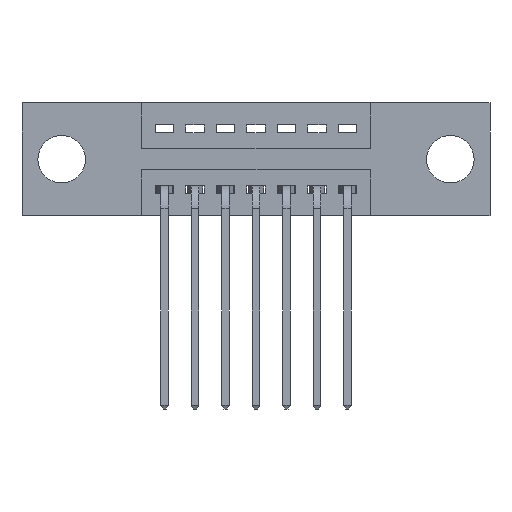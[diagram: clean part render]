
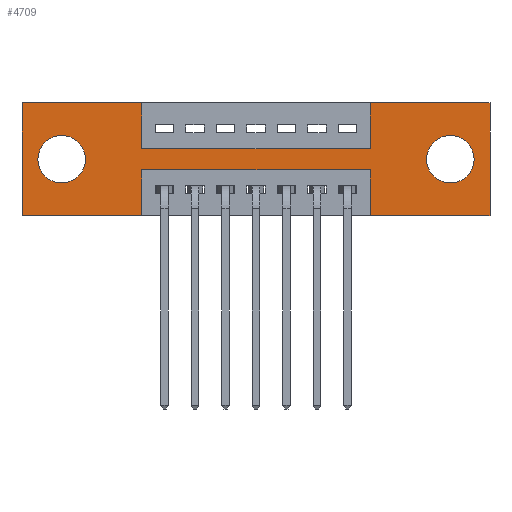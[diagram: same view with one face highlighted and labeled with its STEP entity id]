
A CAD part, front view. The second image highlights one B-rep face of the part: STEP entity #4709.
In plain terms, the highlighted planar face has unit normal (0, -1, 0).
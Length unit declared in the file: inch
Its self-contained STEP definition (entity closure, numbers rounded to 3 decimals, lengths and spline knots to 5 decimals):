
#4 = DIRECTION ( 'NONE',  ( 0., 0., 1. ) ) ;
#67 = ORIENTED_EDGE ( 'NONE', *, *, #2431, .F. ) ;
#70 = ORIENTED_EDGE ( 'NONE', *, *, #4872, .F. ) ;
#92 = ORIENTED_EDGE ( 'NONE', *, *, #8722, .F. ) ;
#132 = ORIENTED_EDGE ( 'NONE', *, *, #4977, .T. ) ;
#203 = ORIENTED_EDGE ( 'NONE', *, *, #1343, .F. ) ;
#391 = ORIENTED_EDGE ( 'NONE', *, *, #4073, .F. ) ;
#434 = CARTESIAN_POINT ( 'NONE',  ( 1.405, 0., -0.107 ) ) ;
#557 = ORIENTED_EDGE ( 'NONE', *, *, #3080, .T. ) ;
#597 = VERTEX_POINT ( 'NONE', #6072 ) ;
#625 = EDGE_CURVE ( 'NONE', #7750, #8362, #4138, .T. ) ;
#644 = VERTEX_POINT ( 'NONE', #993 ) ;
#658 = ORIENTED_EDGE ( 'NONE', *, *, #10028, .F. ) ;
#693 = CARTESIAN_POINT ( 'NONE',  ( 0., 0., -0.37 ) ) ;
#799 = VERTEX_POINT ( 'NONE', #434 ) ;
#810 = EDGE_CURVE ( 'NONE', #5263, #7720, #3069, .T. ) ;
#854 = CARTESIAN_POINT ( 'NONE',  ( 0.13, 0., -0.107 ) ) ;
#937 = VECTOR ( 'NONE', #6131, 39.37008 ) ;
#993 = CARTESIAN_POINT ( 'NONE',  ( 0.3925, 0., -0.37 ) ) ;
#1066 = VECTOR ( 'NONE', #4671, 39.37008 ) ;
#1343 = EDGE_CURVE ( 'NONE', #9410, #3716, #3558, .T. ) ;
#1416 = FACE_OUTER_BOUND ( 'NONE', #4132, .T. ) ;
#1428 = ORIENTED_EDGE ( 'NONE', *, *, #3376, .T. ) ;
#1438 = ORIENTED_EDGE ( 'NONE', *, *, #625, .F. ) ;
#1467 = DIRECTION ( 'NONE',  ( 0., 0., -1. ) ) ;
#1473 = DIRECTION ( 'NONE',  ( 0., 1., 0. ) ) ;
#1483 = CARTESIAN_POINT ( 'NONE',  ( 1.405, 0., -0.185 ) ) ;
#1587 = CARTESIAN_POINT ( 'NONE',  ( 1.535, 0., 0. ) ) ;
#1611 = CARTESIAN_POINT ( 'NONE',  ( 0., 0., -0.37 ) ) ;
#1643 = VERTEX_POINT ( 'NONE', #693 ) ;
#1645 = DIRECTION ( 'NONE',  ( 0., 1., 0. ) ) ;
#1715 = CARTESIAN_POINT ( 'NONE',  ( 0., 0., -0.37 ) ) ;
#1917 = VECTOR ( 'NONE', #8969, 39.37008 ) ;
#2101 = VECTOR ( 'NONE', #2551, 39.37008 ) ;
#2142 = CIRCLE ( 'NONE', #7641, 0.078 ) ;
#2307 = ORIENTED_EDGE ( 'NONE', *, *, #810, .T. ) ;
#2379 = CARTESIAN_POINT ( 'NONE',  ( 0.3925, 0., 0. ) ) ;
#2431 = EDGE_CURVE ( 'NONE', #5848, #7120, #4400, .T. ) ;
#2453 = DIRECTION ( 'NONE',  ( -1., 0., 0. ) ) ;
#2533 = AXIS2_PLACEMENT_3D ( 'NONE', #3192, #3287, #3289 ) ;
#2551 = DIRECTION ( 'NONE',  ( 0., 0., -1. ) ) ;
#2730 = ORIENTED_EDGE ( 'NONE', *, *, #9219, .F. ) ;
#2784 = CIRCLE ( 'NONE', #2533, 0.078 ) ;
#2812 = ORIENTED_EDGE ( 'NONE', *, *, #6426, .F. ) ;
#2928 = ORIENTED_EDGE ( 'NONE', *, *, #8620, .F. ) ;
#3069 = CIRCLE ( 'NONE', #7272, 0.078 ) ;
#3080 = EDGE_CURVE ( 'NONE', #799, #597, #2784, .T. ) ;
#3160 = DIRECTION ( 'NONE',  ( 1., 0., 0. ) ) ;
#3192 = CARTESIAN_POINT ( 'NONE',  ( 1.405, 0., -0.185 ) ) ;
#3262 = LINE ( 'NONE', #9622, #1066 ) ;
#3287 = DIRECTION ( 'NONE',  ( 0., 1., 0. ) ) ;
#3289 = DIRECTION ( 'NONE',  ( 0., 0., -1. ) ) ;
#3376 = EDGE_CURVE ( 'NONE', #7720, #5263, #2142, .T. ) ;
#3449 = DIRECTION ( 'NONE',  ( 0., 0., -1. ) ) ;
#3458 = PLANE ( 'NONE',  #8005 ) ;
#3483 = CARTESIAN_POINT ( 'NONE',  ( 0., 0., -0.37 ) ) ;
#3550 = DIRECTION ( 'NONE',  ( 0., -1., 0. ) ) ;
#3558 = LINE ( 'NONE', #6104, #9057 ) ;
#3716 = VERTEX_POINT ( 'NONE', #4149 ) ;
#3879 = FACE_BOUND ( 'NONE', #3880, .T. ) ;
#3880 = EDGE_LOOP ( 'NONE', ( #557, #132 ) ) ;
#4000 = CARTESIAN_POINT ( 'NONE',  ( 0.3925, 0., -0.15 ) ) ;
#4073 = EDGE_CURVE ( 'NONE', #8362, #644, #9103, .T. ) ;
#4132 = EDGE_LOOP ( 'NONE', ( #391, #1438, #92, #8539, #2730, #67, #8314, #2812, #70, #203, #2928, #658 ) ) ;
#4138 = LINE ( 'NONE', #4354, #1917 ) ;
#4149 = CARTESIAN_POINT ( 'NONE',  ( 0.3925, 0., 0. ) ) ;
#4186 = EDGE_LOOP ( 'NONE', ( #2307, #1428 ) ) ;
#4230 = CARTESIAN_POINT ( 'NONE',  ( 1.1425, 0., 0. ) ) ;
#4323 = VECTOR ( 'NONE', #3160, 39.37008 ) ;
#4354 = CARTESIAN_POINT ( 'NONE',  ( 0.3925, 0., -0.22 ) ) ;
#4400 = LINE ( 'NONE', #6595, #9681 ) ;
#4671 = DIRECTION ( 'NONE',  ( 0., 0., -1. ) ) ;
#4709 = ADVANCED_FACE ( 'NONE', ( #3879, #6087, #1416 ), #3458, .T. ) ;
#4872 = EDGE_CURVE ( 'NONE', #3716, #9176, #8280, .T. ) ;
#4911 = CARTESIAN_POINT ( 'NONE',  ( 0., 0., 0. ) ) ;
#4977 = EDGE_CURVE ( 'NONE', #597, #799, #7218, .T. ) ;
#5263 = VERTEX_POINT ( 'NONE', #854 ) ;
#5353 = CARTESIAN_POINT ( 'NONE',  ( 0., 0., 0. ) ) ;
#5410 = CARTESIAN_POINT ( 'NONE',  ( 0.3925, 0., -0.15 ) ) ;
#5416 = LINE ( 'NONE', #5353, #937 ) ;
#5535 = DIRECTION ( 'NONE',  ( 1., 0., 0. ) ) ;
#5761 = CARTESIAN_POINT ( 'NONE',  ( 0.13, 0., -0.263 ) ) ;
#5792 = CARTESIAN_POINT ( 'NONE',  ( 0.3925, 0., -0.22 ) ) ;
#5848 = VERTEX_POINT ( 'NONE', #4230 ) ;
#5990 = CARTESIAN_POINT ( 'NONE',  ( 1.1425, 0., -0.15 ) ) ;
#5991 = VERTEX_POINT ( 'NONE', #5990 ) ;
#6072 = CARTESIAN_POINT ( 'NONE',  ( 1.405, 0., -0.263 ) ) ;
#6087 = FACE_BOUND ( 'NONE', #4186, .T. ) ;
#6104 = CARTESIAN_POINT ( 'NONE',  ( 0., 0., 0. ) ) ;
#6131 = DIRECTION ( 'NONE',  ( 0., 0., 1. ) ) ;
#6154 = DIRECTION ( 'NONE',  ( 1., 0., 0. ) ) ;
#6426 = EDGE_CURVE ( 'NONE', #9176, #5991, #10036, .T. ) ;
#6427 = AXIS2_PLACEMENT_3D ( 'NONE', #1483, #1473, #1467 ) ;
#6477 = VECTOR ( 'NONE', #8400, 39.37008 ) ;
#6595 = CARTESIAN_POINT ( 'NONE',  ( 0., 0., 0. ) ) ;
#6710 = LINE ( 'NONE', #9605, #6477 ) ;
#7120 = VERTEX_POINT ( 'NONE', #1587 ) ;
#7218 = CIRCLE ( 'NONE', #6427, 0.078 ) ;
#7272 = AXIS2_PLACEMENT_3D ( 'NONE', #9118, #1645, #4 ) ;
#7276 = CARTESIAN_POINT ( 'NONE',  ( 1.535, 0., -0.37 ) ) ;
#7330 = DIRECTION ( 'NONE',  ( -1., 0., 0. ) ) ;
#7362 = VECTOR ( 'NONE', #9241, 39.37008 ) ;
#7411 = VECTOR ( 'NONE', #8667, 39.37008 ) ;
#7584 = CARTESIAN_POINT ( 'NONE',  ( 1.1425, 0., -0.37 ) ) ;
#7627 = LINE ( 'NONE', #10021, #7411 ) ;
#7641 = AXIS2_PLACEMENT_3D ( 'NONE', #9800, #9857, #9892 ) ;
#7720 = VERTEX_POINT ( 'NONE', #5761 ) ;
#7750 = VERTEX_POINT ( 'NONE', #9929 ) ;
#7847 = EDGE_CURVE ( 'NONE', #5991, #5848, #7627, .T. ) ;
#8005 = AXIS2_PLACEMENT_3D ( 'NONE', #3483, #3550, #3449 ) ;
#8018 = VERTEX_POINT ( 'NONE', #7584 ) ;
#8280 = LINE ( 'NONE', #2379, #2101 ) ;
#8314 = ORIENTED_EDGE ( 'NONE', *, *, #7847, .F. ) ;
#8362 = VERTEX_POINT ( 'NONE', #5792 ) ;
#8400 = DIRECTION ( 'NONE',  ( 0., 0., 1. ) ) ;
#8539 = ORIENTED_EDGE ( 'NONE', *, *, #8956, .F. ) ;
#8620 = EDGE_CURVE ( 'NONE', #1643, #9410, #5416, .T. ) ;
#8667 = DIRECTION ( 'NONE',  ( 0., 0., 1. ) ) ;
#8722 = EDGE_CURVE ( 'NONE', #8018, #7750, #6710, .T. ) ;
#8956 = EDGE_CURVE ( 'NONE', #10078, #8018, #9769, .T. ) ;
#8969 = DIRECTION ( 'NONE',  ( -1., 0., 0. ) ) ;
#9057 = VECTOR ( 'NONE', #6154, 39.37008 ) ;
#9103 = LINE ( 'NONE', #9197, #7362 ) ;
#9118 = CARTESIAN_POINT ( 'NONE',  ( 0.13, 0., -0.185 ) ) ;
#9176 = VERTEX_POINT ( 'NONE', #5410 ) ;
#9197 = CARTESIAN_POINT ( 'NONE',  ( 0.3925, 0., -0.37 ) ) ;
#9219 = EDGE_CURVE ( 'NONE', #7120, #10078, #3262, .T. ) ;
#9241 = DIRECTION ( 'NONE',  ( 0., 0., -1. ) ) ;
#9410 = VERTEX_POINT ( 'NONE', #4911 ) ;
#9605 = CARTESIAN_POINT ( 'NONE',  ( 1.1425, 0., -0.37 ) ) ;
#9622 = CARTESIAN_POINT ( 'NONE',  ( 1.535, 0., 0. ) ) ;
#9681 = VECTOR ( 'NONE', #5535, 39.37008 ) ;
#9747 = VECTOR ( 'NONE', #2453, 39.37008 ) ;
#9769 = LINE ( 'NONE', #1715, #9984 ) ;
#9800 = CARTESIAN_POINT ( 'NONE',  ( 0.13, 0., -0.185 ) ) ;
#9857 = DIRECTION ( 'NONE',  ( 0., 1., 0. ) ) ;
#9892 = DIRECTION ( 'NONE',  ( 0., 0., 1. ) ) ;
#9929 = CARTESIAN_POINT ( 'NONE',  ( 1.1425, 0., -0.22 ) ) ;
#9959 = LINE ( 'NONE', #1611, #9747 ) ;
#9984 = VECTOR ( 'NONE', #7330, 39.37008 ) ;
#10021 = CARTESIAN_POINT ( 'NONE',  ( 1.1425, 0., 0. ) ) ;
#10028 = EDGE_CURVE ( 'NONE', #644, #1643, #9959, .T. ) ;
#10036 = LINE ( 'NONE', #4000, #4323 ) ;
#10078 = VERTEX_POINT ( 'NONE', #7276 ) ;
